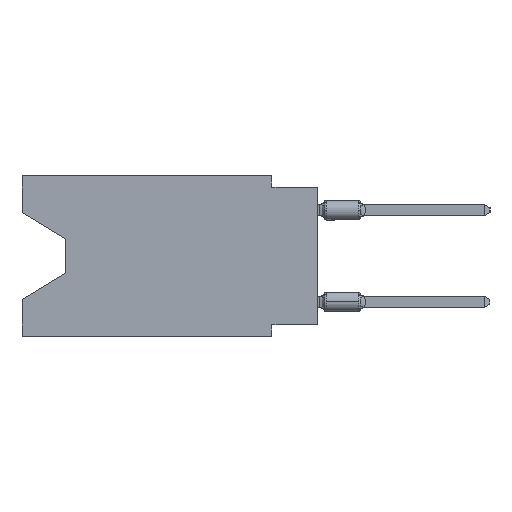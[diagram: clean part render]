
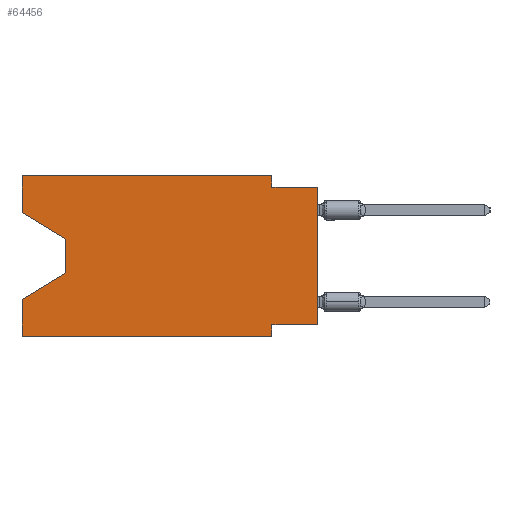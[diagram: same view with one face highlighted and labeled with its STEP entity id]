
A CAD part, left-side view. The second image highlights one B-rep face of the part: STEP entity #64456.
In plain terms, the highlighted planar face has unit normal (-1, 0, 0).
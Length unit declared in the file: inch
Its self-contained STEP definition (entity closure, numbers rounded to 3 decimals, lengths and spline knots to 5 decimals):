
#705 = VERTEX_POINT ( 'NONE', #16869 ) ;
#1109 = LINE ( 'NONE', #28565, #65021 ) ;
#1219 = LINE ( 'NONE', #21994, #15128 ) ;
#1567 = DIRECTION ( 'NONE',  ( 0., 0., -1. ) ) ;
#1941 = VECTOR ( 'NONE', #35858, 39.37008 ) ;
#3197 = LINE ( 'NONE', #23620, #66690 ) ;
#4040 = VECTOR ( 'NONE', #63362, 39.37008 ) ;
#5167 = CARTESIAN_POINT ( 'NONE',  ( 0., 0.645, 0. ) ) ;
#5697 = EDGE_CURVE ( 'NONE', #24828, #55309, #46499, .T. ) ;
#7097 = CARTESIAN_POINT ( 'NONE',  ( 0., 0., -0.325 ) ) ;
#7330 = DIRECTION ( 'NONE',  ( 1., 0., 0. ) ) ;
#7969 = VECTOR ( 'NONE', #15841, 39.37008 ) ;
#9313 = LINE ( 'NONE', #25004, #52931 ) ;
#9418 = VECTOR ( 'NONE', #46830, 39.37008 ) ;
#10987 = ORIENTED_EDGE ( 'NONE', *, *, #44178, .F. ) ;
#11441 = CARTESIAN_POINT ( 'NONE',  ( 0., 0.645, 0. ) ) ;
#12425 = PLANE ( 'NONE',  #39725 ) ;
#12524 = LINE ( 'NONE', #7097, #34437 ) ;
#12916 = EDGE_CURVE ( 'NONE', #43172, #47954, #3197, .T. ) ;
#13375 = EDGE_LOOP ( 'NONE', ( #31156, #39595, #66935, #29847, #59042, #33397, #47949, #31290, #21211, #24965, #10987, #27789 ) ) ;
#15057 = LINE ( 'NONE', #5167, #1941 ) ;
#15128 = VECTOR ( 'NONE', #16885, 39.37008 ) ;
#15841 = DIRECTION ( 'NONE',  ( 0., -0.855, -0.519 ) ) ;
#16869 = CARTESIAN_POINT ( 'NONE',  ( 0., 0.55, -0.212 ) ) ;
#16885 = DIRECTION ( 'NONE',  ( 0., 0., 1. ) ) ;
#16996 = LINE ( 'NONE', #42576, #4040 ) ;
#18089 = CARTESIAN_POINT ( 'NONE',  ( 0., 0.1, -0.325 ) ) ;
#18240 = FACE_OUTER_BOUND ( 'NONE', #13375, .T. ) ;
#19629 = VERTEX_POINT ( 'NONE', #35449 ) ;
#20916 = LINE ( 'NONE', #50932, #9418 ) ;
#21211 = ORIENTED_EDGE ( 'NONE', *, *, #58278, .F. ) ;
#21994 = CARTESIAN_POINT ( 'NONE',  ( 0., 0.645, 0. ) ) ;
#22095 = VERTEX_POINT ( 'NONE', #18089 ) ;
#22972 = CARTESIAN_POINT ( 'NONE',  ( 0., 0.645, -0.35 ) ) ;
#23620 = CARTESIAN_POINT ( 'NONE',  ( 0., 0., 0. ) ) ;
#24505 = EDGE_CURVE ( 'NONE', #24828, #26930, #1219, .T. ) ;
#24828 = VERTEX_POINT ( 'NONE', #36871 ) ;
#24917 = VERTEX_POINT ( 'NONE', #27273 ) ;
#24965 = ORIENTED_EDGE ( 'NONE', *, *, #38769, .F. ) ;
#25004 = CARTESIAN_POINT ( 'NONE',  ( 0., 0.1, 0. ) ) ;
#26683 = CARTESIAN_POINT ( 'NONE',  ( 0., 0.645, 0. ) ) ;
#26930 = VERTEX_POINT ( 'NONE', #11441 ) ;
#27273 = CARTESIAN_POINT ( 'NONE',  ( 0., 0.1, -0.35 ) ) ;
#27789 = ORIENTED_EDGE ( 'NONE', *, *, #24505, .F. ) ;
#27812 = VECTOR ( 'NONE', #51366, 39.37008 ) ;
#27866 = DIRECTION ( 'NONE',  ( 0., 1., 0. ) ) ;
#28565 = CARTESIAN_POINT ( 'NONE',  ( 0., 0., -0.025 ) ) ;
#29376 = VECTOR ( 'NONE', #31866, 39.37008 ) ;
#29847 = ORIENTED_EDGE ( 'NONE', *, *, #42396, .F. ) ;
#29944 = CARTESIAN_POINT ( 'NONE',  ( 0., 0.1, 0. ) ) ;
#30138 = EDGE_CURVE ( 'NONE', #42491, #24917, #20916, .T. ) ;
#30563 = CARTESIAN_POINT ( 'NONE',  ( 0., 0.55, -0.212 ) ) ;
#31156 = ORIENTED_EDGE ( 'NONE', *, *, #5697, .T. ) ;
#31290 = ORIENTED_EDGE ( 'NONE', *, *, #12916, .T. ) ;
#31866 = DIRECTION ( 'NONE',  ( 0., 0., -1. ) ) ;
#33397 = ORIENTED_EDGE ( 'NONE', *, *, #56936, .F. ) ;
#33509 = DIRECTION ( 'NONE',  ( 0., 0., 1. ) ) ;
#34437 = VECTOR ( 'NONE', #27866, 39.37008 ) ;
#35449 = CARTESIAN_POINT ( 'NONE',  ( 0., 0.645, -0.26975 ) ) ;
#35858 = DIRECTION ( 'NONE',  ( 0., 0., 1. ) ) ;
#36620 = CARTESIAN_POINT ( 'NONE',  ( 0., 0.645, -0.08025 ) ) ;
#36871 = CARTESIAN_POINT ( 'NONE',  ( 0., 0.645, -0.08025 ) ) ;
#37008 = LINE ( 'NONE', #57766, #29376 ) ;
#38769 = EDGE_CURVE ( 'NONE', #67375, #63381, #9313, .T. ) ;
#39595 = ORIENTED_EDGE ( 'NONE', *, *, #44752, .T. ) ;
#39725 = AXIS2_PLACEMENT_3D ( 'NONE', #53670, #7330, #1567 ) ;
#40804 = LINE ( 'NONE', #30563, #27812 ) ;
#41683 = LINE ( 'NONE', #26683, #54305 ) ;
#42396 = EDGE_CURVE ( 'NONE', #42491, #19629, #15057, .T. ) ;
#42491 = VERTEX_POINT ( 'NONE', #22972 ) ;
#42576 = CARTESIAN_POINT ( 'NONE',  ( 0., 0.1, -0.35 ) ) ;
#43172 = VERTEX_POINT ( 'NONE', #48434 ) ;
#44178 = EDGE_CURVE ( 'NONE', #26930, #67375, #41683, .T. ) ;
#44499 = CARTESIAN_POINT ( 'NONE',  ( 0., 0.55, -0.138 ) ) ;
#44752 = EDGE_CURVE ( 'NONE', #55309, #705, #37008, .T. ) ;
#46499 = LINE ( 'NONE', #36620, #7969 ) ;
#46830 = DIRECTION ( 'NONE',  ( 0., -1., 0. ) ) ;
#47949 = ORIENTED_EDGE ( 'NONE', *, *, #54844, .F. ) ;
#47954 = VERTEX_POINT ( 'NONE', #64049 ) ;
#48093 = DIRECTION ( 'NONE',  ( 0., -1., 0. ) ) ;
#48434 = CARTESIAN_POINT ( 'NONE',  ( 0., 0., -0.325 ) ) ;
#50529 = CARTESIAN_POINT ( 'NONE',  ( 0., 0.1, -0.025 ) ) ;
#50932 = CARTESIAN_POINT ( 'NONE',  ( 0., 0.645, -0.35 ) ) ;
#51248 = DIRECTION ( 'NONE',  ( 0., 0., -1. ) ) ;
#51366 = DIRECTION ( 'NONE',  ( 0., 0.855, -0.519 ) ) ;
#52931 = VECTOR ( 'NONE', #51248, 39.37008 ) ;
#53670 = CARTESIAN_POINT ( 'NONE',  ( 0., 0.645, 0. ) ) ;
#54305 = VECTOR ( 'NONE', #58020, 39.37008 ) ;
#54844 = EDGE_CURVE ( 'NONE', #43172, #22095, #12524, .T. ) ;
#55309 = VERTEX_POINT ( 'NONE', #44499 ) ;
#56936 = EDGE_CURVE ( 'NONE', #22095, #24917, #16996, .T. ) ;
#57766 = CARTESIAN_POINT ( 'NONE',  ( 0., 0.55, -0.138 ) ) ;
#58020 = DIRECTION ( 'NONE',  ( 0., -1., 0. ) ) ;
#58278 = EDGE_CURVE ( 'NONE', #63381, #47954, #1109, .T. ) ;
#59042 = ORIENTED_EDGE ( 'NONE', *, *, #30138, .T. ) ;
#63362 = DIRECTION ( 'NONE',  ( 0., 0., -1. ) ) ;
#63381 = VERTEX_POINT ( 'NONE', #50529 ) ;
#64049 = CARTESIAN_POINT ( 'NONE',  ( 0., 0., -0.025 ) ) ;
#64456 = ADVANCED_FACE ( 'NONE', ( #18240 ), #12425, .F. ) ;
#65021 = VECTOR ( 'NONE', #48093, 39.37008 ) ;
#65522 = EDGE_CURVE ( 'NONE', #705, #19629, #40804, .T. ) ;
#66690 = VECTOR ( 'NONE', #33509, 39.37008 ) ;
#66935 = ORIENTED_EDGE ( 'NONE', *, *, #65522, .T. ) ;
#67375 = VERTEX_POINT ( 'NONE', #29944 ) ;
